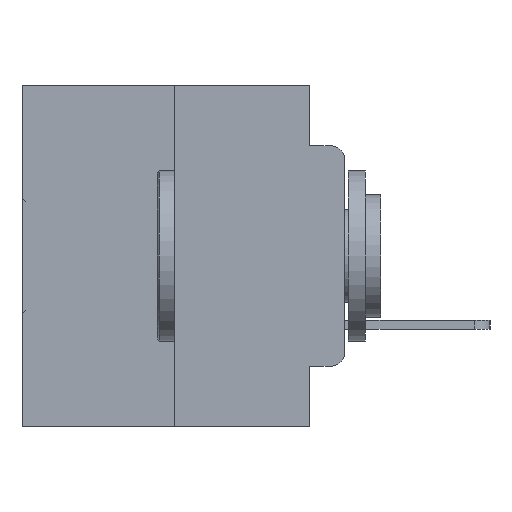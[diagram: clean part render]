
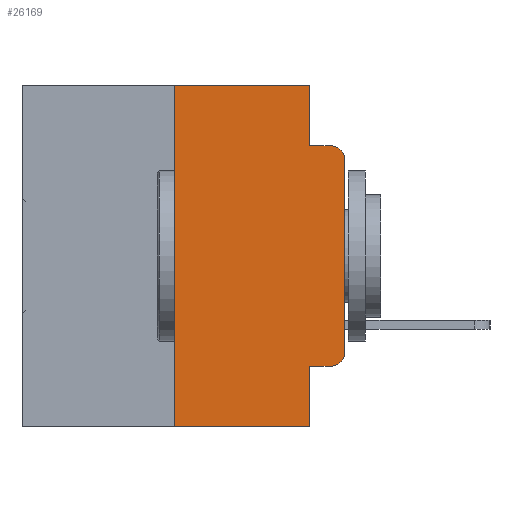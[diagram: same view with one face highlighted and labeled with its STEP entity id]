
A CAD part, left-side view. The second image highlights one B-rep face of the part: STEP entity #26169.
In plain terms, the highlighted planar face has unit normal (-1, 0, 0).
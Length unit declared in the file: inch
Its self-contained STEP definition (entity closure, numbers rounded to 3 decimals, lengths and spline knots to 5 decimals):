
#230 = VERTEX_POINT ( 'NONE', #22292 ) ;
#281 = VECTOR ( 'NONE', #4684, 39.37008 ) ;
#511 = CARTESIAN_POINT ( 'NONE',  ( 0., 0.02, -0.1085 ) ) ;
#976 = DIRECTION ( 'NONE',  ( 0., 0., -1. ) ) ;
#2528 = CARTESIAN_POINT ( 'NONE',  ( 0., 0.473, 0. ) ) ;
#2649 = VERTEX_POINT ( 'NONE', #27033 ) ;
#3272 = CARTESIAN_POINT ( 'NONE',  ( 0., 0.25, -0.5 ) ) ;
#4208 = VECTOR ( 'NONE', #24898, 39.37008 ) ;
#4684 = DIRECTION ( 'NONE',  ( 0., -1., 0. ) ) ;
#5431 = LINE ( 'NONE', #6393, #24012 ) ;
#5662 = ORIENTED_EDGE ( 'NONE', *, *, #9307, .F. ) ;
#6393 = CARTESIAN_POINT ( 'NONE',  ( 0., 0.051, 0. ) ) ;
#6491 = CARTESIAN_POINT ( 'NONE',  ( 0., 0.051, -0.0885 ) ) ;
#6985 = CARTESIAN_POINT ( 'NONE',  ( 0., 0.473, 0. ) ) ;
#7249 = ORIENTED_EDGE ( 'NONE', *, *, #15702, .T. ) ;
#8372 = ORIENTED_EDGE ( 'NONE', *, *, #31541, .T. ) ;
#8570 = CARTESIAN_POINT ( 'NONE',  ( 0., 0.02, -0.3915 ) ) ;
#9307 = EDGE_CURVE ( 'NONE', #24705, #10741, #29115, .T. ) ;
#10003 = VERTEX_POINT ( 'NONE', #16334 ) ;
#10741 = VERTEX_POINT ( 'NONE', #24647 ) ;
#10805 = ORIENTED_EDGE ( 'NONE', *, *, #17952, .F. ) ;
#10812 = VERTEX_POINT ( 'NONE', #17595 ) ;
#11074 = ORIENTED_EDGE ( 'NONE', *, *, #15271, .F. ) ;
#11243 = VECTOR ( 'NONE', #17023, 39.37008 ) ;
#11254 = ORIENTED_EDGE ( 'NONE', *, *, #31072, .T. ) ;
#11291 = DIRECTION ( 'NONE',  ( 0., -1., 0. ) ) ;
#11626 = CARTESIAN_POINT ( 'NONE',  ( 0., 0.051, -0.0885 ) ) ;
#11641 = CARTESIAN_POINT ( 'NONE',  ( 0., 0., -0.1085 ) ) ;
#12090 = LINE ( 'NONE', #29399, #11243 ) ;
#12160 = LINE ( 'NONE', #6985, #281 ) ;
#12381 = AXIS2_PLACEMENT_3D ( 'NONE', #511, #23484, #30842 ) ;
#12419 = LINE ( 'NONE', #20503, #31723 ) ;
#13235 = VERTEX_POINT ( 'NONE', #19426 ) ;
#14416 = CIRCLE ( 'NONE', #12381, 0.02 ) ;
#14817 = DIRECTION ( 'NONE',  ( 1., 0., 0. ) ) ;
#15080 = EDGE_CURVE ( 'NONE', #13235, #230, #5431, .T. ) ;
#15083 = CARTESIAN_POINT ( 'NONE',  ( 0., 0.473, -0.5 ) ) ;
#15087 = CARTESIAN_POINT ( 'NONE',  ( 0., 0., 0. ) ) ;
#15271 = EDGE_CURVE ( 'NONE', #16087, #10812, #12160, .T. ) ;
#15702 = EDGE_CURVE ( 'NONE', #2649, #20499, #17253, .T. ) ;
#16087 = VERTEX_POINT ( 'NONE', #19454 ) ;
#16163 = LINE ( 'NONE', #19693, #31111 ) ;
#16334 = CARTESIAN_POINT ( 'NONE',  ( 0., 0.02, -0.4115 ) ) ;
#17023 = DIRECTION ( 'NONE',  ( 0., 0., 1. ) ) ;
#17253 = LINE ( 'NONE', #15087, #23566 ) ;
#17315 = VERTEX_POINT ( 'NONE', #3272 ) ;
#17455 = PLANE ( 'NONE',  #22809 ) ;
#17595 = CARTESIAN_POINT ( 'NONE',  ( 0., 0.051, 0. ) ) ;
#17952 = EDGE_CURVE ( 'NONE', #10812, #24705, #16163, .T. ) ;
#18470 = ORIENTED_EDGE ( 'NONE', *, *, #32344, .T. ) ;
#19426 = CARTESIAN_POINT ( 'NONE',  ( 0., 0.051, -0.4115 ) ) ;
#19454 = CARTESIAN_POINT ( 'NONE',  ( 0., 0.25, 0. ) ) ;
#19693 = CARTESIAN_POINT ( 'NONE',  ( 0., 0.051, 0. ) ) ;
#20499 = VERTEX_POINT ( 'NONE', #11641 ) ;
#20503 = CARTESIAN_POINT ( 'NONE',  ( 0., 0.051, -0.4115 ) ) ;
#20536 = EDGE_CURVE ( 'NONE', #17315, #16087, #12090, .T. ) ;
#20988 = DIRECTION ( 'NONE',  ( 0., 0., -1. ) ) ;
#21199 = ORIENTED_EDGE ( 'NONE', *, *, #26842, .T. ) ;
#21248 = FACE_OUTER_BOUND ( 'NONE', #32237, .T. ) ;
#21910 = ORIENTED_EDGE ( 'NONE', *, *, #20536, .F. ) ;
#22292 = CARTESIAN_POINT ( 'NONE',  ( 0., 0.051, -0.5 ) ) ;
#22809 = AXIS2_PLACEMENT_3D ( 'NONE', #2528, #14817, #30029 ) ;
#23484 = DIRECTION ( 'NONE',  ( -1., 0., 0. ) ) ;
#23500 = DIRECTION ( 'NONE',  ( -1., 0., 0. ) ) ;
#23566 = VECTOR ( 'NONE', #27242, 39.37008 ) ;
#24012 = VECTOR ( 'NONE', #976, 39.37008 ) ;
#24590 = AXIS2_PLACEMENT_3D ( 'NONE', #8570, #23500, #20988 ) ;
#24647 = CARTESIAN_POINT ( 'NONE',  ( 0., 0.02, -0.0885 ) ) ;
#24705 = VERTEX_POINT ( 'NONE', #6491 ) ;
#24898 = DIRECTION ( 'NONE',  ( 0., -1., 0. ) ) ;
#26169 = ADVANCED_FACE ( 'NONE', ( #21248 ), #17455, .F. ) ;
#26842 = EDGE_CURVE ( 'NONE', #17315, #230, #28261, .T. ) ;
#27033 = CARTESIAN_POINT ( 'NONE',  ( 0., 0., -0.3915 ) ) ;
#27242 = DIRECTION ( 'NONE',  ( 0., 0., 1. ) ) ;
#28261 = LINE ( 'NONE', #15083, #4208 ) ;
#29115 = LINE ( 'NONE', #11626, #31424 ) ;
#29399 = CARTESIAN_POINT ( 'NONE',  ( 0., 0.25, 0. ) ) ;
#29923 = DIRECTION ( 'NONE',  ( 0., 0., -1. ) ) ;
#30029 = DIRECTION ( 'NONE',  ( 0., 0., -1. ) ) ;
#30113 = DIRECTION ( 'NONE',  ( 0., -1., 0. ) ) ;
#30756 = ORIENTED_EDGE ( 'NONE', *, *, #15080, .F. ) ;
#30842 = DIRECTION ( 'NONE',  ( 0., 0., -1. ) ) ;
#31072 = EDGE_CURVE ( 'NONE', #10003, #2649, #31757, .T. ) ;
#31111 = VECTOR ( 'NONE', #29923, 39.37008 ) ;
#31424 = VECTOR ( 'NONE', #11291, 39.37008 ) ;
#31541 = EDGE_CURVE ( 'NONE', #13235, #10003, #12419, .T. ) ;
#31723 = VECTOR ( 'NONE', #30113, 39.37008 ) ;
#31757 = CIRCLE ( 'NONE', #24590, 0.02 ) ;
#32237 = EDGE_LOOP ( 'NONE', ( #7249, #18470, #5662, #10805, #11074, #21910, #21199, #30756, #8372, #11254 ) ) ;
#32344 = EDGE_CURVE ( 'NONE', #20499, #10741, #14416, .T. ) ;
